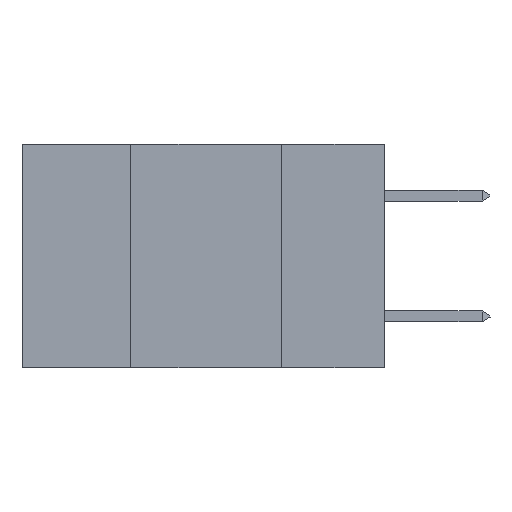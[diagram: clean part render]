
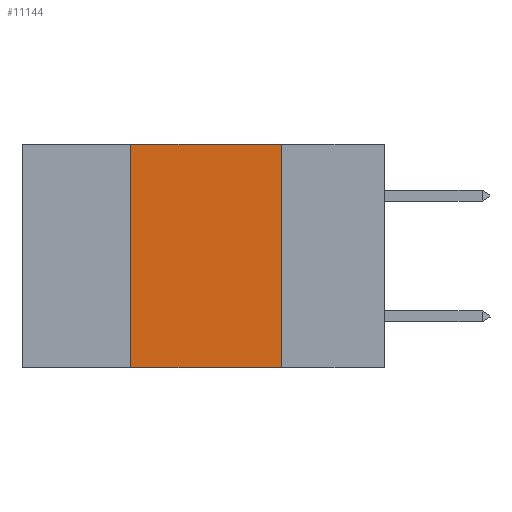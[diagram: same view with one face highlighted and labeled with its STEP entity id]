
A CAD part, left-side view. The second image highlights one B-rep face of the part: STEP entity #11144.
In plain terms, the highlighted planar face has unit normal (-1, 0, 0).
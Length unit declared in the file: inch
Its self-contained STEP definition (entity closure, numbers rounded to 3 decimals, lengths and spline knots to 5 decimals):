
#1277 = FACE_OUTER_BOUND ( 'NONE', #7257, .T. ) ;
#1899 = CARTESIAN_POINT ( 'NONE',  ( 0., 0.17, 0. ) ) ;
#2486 = LINE ( 'NONE', #10033, #19623 ) ;
#2632 = DIRECTION ( 'NONE',  ( 0., 0., 1. ) ) ;
#3433 = EDGE_CURVE ( 'NONE', #35227, #31437, #2486, .T. ) ;
#4760 = ORIENTED_EDGE ( 'NONE', *, *, #10772, .T. ) ;
#4870 = VECTOR ( 'NONE', #16499, 39.37008 ) ;
#6862 = CARTESIAN_POINT ( 'NONE',  ( 0., 0.42, -0.37 ) ) ;
#7257 = EDGE_LOOP ( 'NONE', ( #31372, #10427, #26503, #4760 ) ) ;
#8681 = LINE ( 'NONE', #24979, #13098 ) ;
#9330 = DIRECTION ( 'NONE',  ( 0., 0., -1. ) ) ;
#9907 = DIRECTION ( 'NONE',  ( 0., -1., 0. ) ) ;
#9919 = CARTESIAN_POINT ( 'NONE',  ( 0., 0.42, 0. ) ) ;
#10033 = CARTESIAN_POINT ( 'NONE',  ( 0., 0.6, 0. ) ) ;
#10093 = CARTESIAN_POINT ( 'NONE',  ( 0., 0.6, 0. ) ) ;
#10427 = ORIENTED_EDGE ( 'NONE', *, *, #3433, .F. ) ;
#10638 = CARTESIAN_POINT ( 'NONE',  ( 0., 0.17, -0.37 ) ) ;
#10772 = EDGE_CURVE ( 'NONE', #33825, #35251, #15367, .T. ) ;
#11144 = ADVANCED_FACE ( 'NONE', ( #1277 ), #18470, .F. ) ;
#12598 = VECTOR ( 'NONE', #9330, 39.37008 ) ;
#13098 = VECTOR ( 'NONE', #2632, 39.37008 ) ;
#15367 = LINE ( 'NONE', #16973, #4870 ) ;
#16499 = DIRECTION ( 'NONE',  ( 0., -1., 0. ) ) ;
#16543 = LINE ( 'NONE', #23234, #12598 ) ;
#16973 = CARTESIAN_POINT ( 'NONE',  ( 0., 0.6, -0.37 ) ) ;
#18470 = PLANE ( 'NONE',  #20631 ) ;
#19623 = VECTOR ( 'NONE', #9907, 39.37008 ) ;
#20631 = AXIS2_PLACEMENT_3D ( 'NONE', #10093, #29756, #24708 ) ;
#23234 = CARTESIAN_POINT ( 'NONE',  ( 0., 0.17, 0. ) ) ;
#23944 = EDGE_CURVE ( 'NONE', #33825, #35227, #8681, .T. ) ;
#24708 = DIRECTION ( 'NONE',  ( 0., 0., -1. ) ) ;
#24979 = CARTESIAN_POINT ( 'NONE',  ( 0., 0.42, 0. ) ) ;
#25481 = EDGE_CURVE ( 'NONE', #31437, #35251, #16543, .T. ) ;
#26503 = ORIENTED_EDGE ( 'NONE', *, *, #23944, .F. ) ;
#29756 = DIRECTION ( 'NONE',  ( 1., 0., 0. ) ) ;
#31372 = ORIENTED_EDGE ( 'NONE', *, *, #25481, .F. ) ;
#31437 = VERTEX_POINT ( 'NONE', #1899 ) ;
#33825 = VERTEX_POINT ( 'NONE', #6862 ) ;
#35227 = VERTEX_POINT ( 'NONE', #9919 ) ;
#35251 = VERTEX_POINT ( 'NONE', #10638 ) ;
